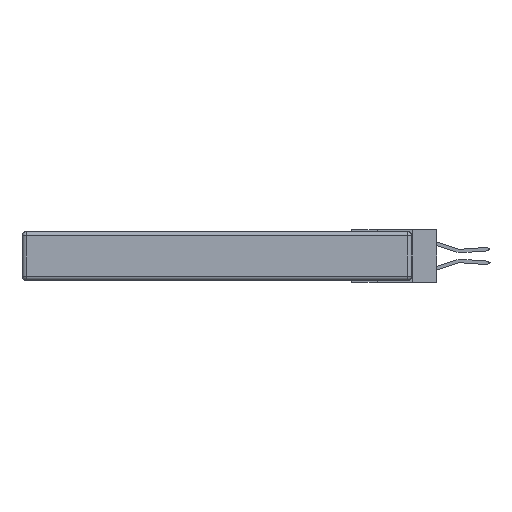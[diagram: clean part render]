
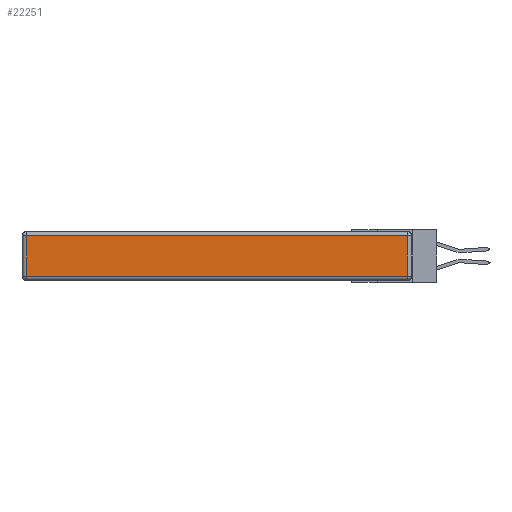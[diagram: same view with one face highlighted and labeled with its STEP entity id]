
A CAD part, left-side view. The second image highlights one B-rep face of the part: STEP entity #22251.
In plain terms, the highlighted planar face has unit normal (-1, 0, 0).
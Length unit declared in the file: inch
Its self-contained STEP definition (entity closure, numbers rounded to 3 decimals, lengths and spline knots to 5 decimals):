
#120 = ORIENTED_EDGE ( 'NONE', *, *, #5615, .T. ) ;
#535 = VECTOR ( 'NONE', #11786, 39.37008 ) ;
#1622 = DIRECTION ( 'NONE',  ( 0., 0., -1. ) ) ;
#1961 = CARTESIAN_POINT ( 'NONE',  ( 0., 2.72, -0.343 ) ) ;
#2058 = DIRECTION ( 'NONE',  ( -1., 0., 0. ) ) ;
#2922 = VERTEX_POINT ( 'NONE', #13330 ) ;
#5615 = EDGE_CURVE ( 'NONE', #2922, #23842, #6823, .T. ) ;
#6823 = LINE ( 'NONE', #1961, #21385 ) ;
#7186 = EDGE_CURVE ( 'NONE', #13086, #17889, #14239, .T. ) ;
#7530 = ORIENTED_EDGE ( 'NONE', *, *, #23407, .T. ) ;
#7676 = CARTESIAN_POINT ( 'NONE',  ( 0., 0.03, -0.313 ) ) ;
#7768 = PLANE ( 'NONE',  #8061 ) ;
#7975 = DIRECTION ( 'NONE',  ( 0., 1., 0. ) ) ;
#8061 = AXIS2_PLACEMENT_3D ( 'NONE', #22952, #2058, #20796 ) ;
#8083 = VECTOR ( 'NONE', #11115, 39.37008 ) ;
#8380 = ORIENTED_EDGE ( 'NONE', *, *, #10964, .T. ) ;
#8649 = ORIENTED_EDGE ( 'NONE', *, *, #7186, .T. ) ;
#10478 = LINE ( 'NONE', #20303, #8083 ) ;
#10964 = EDGE_CURVE ( 'NONE', #17889, #2922, #23300, .T. ) ;
#11115 = DIRECTION ( 'NONE',  ( 0., -1., 0. ) ) ;
#11786 = DIRECTION ( 'NONE',  ( 0., 0., 1. ) ) ;
#12224 = CARTESIAN_POINT ( 'NONE',  ( 0., 2.72, -0.313 ) ) ;
#12909 = FACE_OUTER_BOUND ( 'NONE', #13363, .T. ) ;
#13086 = VERTEX_POINT ( 'NONE', #7676 ) ;
#13330 = CARTESIAN_POINT ( 'NONE',  ( 0., 2.72, -0.03 ) ) ;
#13363 = EDGE_LOOP ( 'NONE', ( #7530, #8649, #8380, #120 ) ) ;
#13667 = CARTESIAN_POINT ( 'NONE',  ( 0., 2.75, -0.03 ) ) ;
#14239 = LINE ( 'NONE', #24419, #535 ) ;
#17019 = CARTESIAN_POINT ( 'NONE',  ( 0., 0.03, -0.03 ) ) ;
#17889 = VERTEX_POINT ( 'NONE', #17019 ) ;
#20303 = CARTESIAN_POINT ( 'NONE',  ( 0., 0., -0.313 ) ) ;
#20796 = DIRECTION ( 'NONE',  ( 0., 0., 1. ) ) ;
#21385 = VECTOR ( 'NONE', #1622, 39.37008 ) ;
#22251 = ADVANCED_FACE ( 'NONE', ( #12909 ), #7768, .T. ) ;
#22952 = CARTESIAN_POINT ( 'NONE',  ( 0., 0., -0.343 ) ) ;
#23300 = LINE ( 'NONE', #13667, #23591 ) ;
#23407 = EDGE_CURVE ( 'NONE', #23842, #13086, #10478, .T. ) ;
#23591 = VECTOR ( 'NONE', #7975, 39.37008 ) ;
#23842 = VERTEX_POINT ( 'NONE', #12224 ) ;
#24419 = CARTESIAN_POINT ( 'NONE',  ( 0., 0.03, -0.343 ) ) ;
